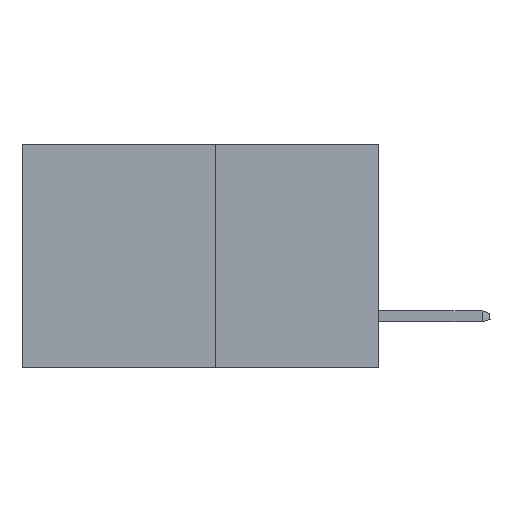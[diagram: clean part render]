
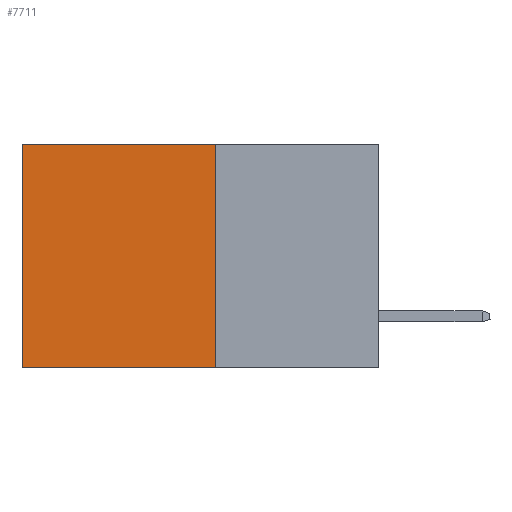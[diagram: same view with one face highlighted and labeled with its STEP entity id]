
A CAD part, left-side view. The second image highlights one B-rep face of the part: STEP entity #7711.
In plain terms, the highlighted planar face has unit normal (-1, 0, 0).
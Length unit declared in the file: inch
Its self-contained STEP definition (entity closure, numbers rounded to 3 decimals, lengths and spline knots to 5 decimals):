
#641 = CARTESIAN_POINT ( 'NONE',  ( 0.277, 0.27, -0.37 ) ) ;
#756 = CARTESIAN_POINT ( 'NONE',  ( 0.277, 0.27, 0. ) ) ;
#1046 = VERTEX_POINT ( 'NONE', #12491 ) ;
#1543 = VECTOR ( 'NONE', #11918, 39.37008 ) ;
#2089 = VECTOR ( 'NONE', #4119, 39.37008 ) ;
#3579 = VERTEX_POINT ( 'NONE', #756 ) ;
#3623 = EDGE_LOOP ( 'NONE', ( #4266, #4314, #4420, #4615 ) ) ;
#4105 = EDGE_CURVE ( 'NONE', #3579, #1046, #14037, .T. ) ;
#4119 = DIRECTION ( 'NONE',  ( 0., 1., 0. ) ) ;
#4266 = ORIENTED_EDGE ( 'NONE', *, *, #14288, .T. ) ;
#4314 = ORIENTED_EDGE ( 'NONE', *, *, #7560, .F. ) ;
#4414 = CARTESIAN_POINT ( 'NONE',  ( 0.277, 0.27, 0. ) ) ;
#4420 = ORIENTED_EDGE ( 'NONE', *, *, #14395, .F. ) ;
#4615 = ORIENTED_EDGE ( 'NONE', *, *, #4105, .T. ) ;
#4805 = LINE ( 'NONE', #11872, #1543 ) ;
#5863 = VERTEX_POINT ( 'NONE', #11848 ) ;
#6299 = CARTESIAN_POINT ( 'NONE',  ( 0.277, 0.59, -0.37 ) ) ;
#6745 = VECTOR ( 'NONE', #9970, 39.37008 ) ;
#7560 = EDGE_CURVE ( 'NONE', #5863, #14239, #12002, .T. ) ;
#7711 = ADVANCED_FACE ( 'NONE', ( #12490 ), #14302, .F. ) ;
#9970 = DIRECTION ( 'NONE',  ( 0., 0., -1. ) ) ;
#10092 = AXIS2_PLACEMENT_3D ( 'NONE', #14343, #14227, #14211 ) ;
#11662 = VECTOR ( 'NONE', #14506, 39.37008 ) ;
#11848 = CARTESIAN_POINT ( 'NONE',  ( 0.277, 0.27, -0.37 ) ) ;
#11872 = CARTESIAN_POINT ( 'NONE',  ( 0.277, 0.59, -0.37 ) ) ;
#11918 = DIRECTION ( 'NONE',  ( 0., 0., -1. ) ) ;
#12002 = LINE ( 'NONE', #14472, #11662 ) ;
#12490 = FACE_OUTER_BOUND ( 'NONE', #3623, .T. ) ;
#12491 = CARTESIAN_POINT ( 'NONE',  ( 0.277, 0.59, 0. ) ) ;
#14037 = LINE ( 'NONE', #4414, #2089 ) ;
#14211 = DIRECTION ( 'NONE',  ( 0., 0., -1. ) ) ;
#14227 = DIRECTION ( 'NONE',  ( 1., 0., 0. ) ) ;
#14239 = VERTEX_POINT ( 'NONE', #6299 ) ;
#14288 = EDGE_CURVE ( 'NONE', #1046, #14239, #4805, .T. ) ;
#14302 = PLANE ( 'NONE',  #10092 ) ;
#14343 = CARTESIAN_POINT ( 'NONE',  ( 0.277, 0.27, -0.37 ) ) ;
#14395 = EDGE_CURVE ( 'NONE', #3579, #5863, #14678, .T. ) ;
#14472 = CARTESIAN_POINT ( 'NONE',  ( 0.277, 0.27, -0.37 ) ) ;
#14506 = DIRECTION ( 'NONE',  ( 0., 1., 0. ) ) ;
#14678 = LINE ( 'NONE', #641, #6745 ) ;
